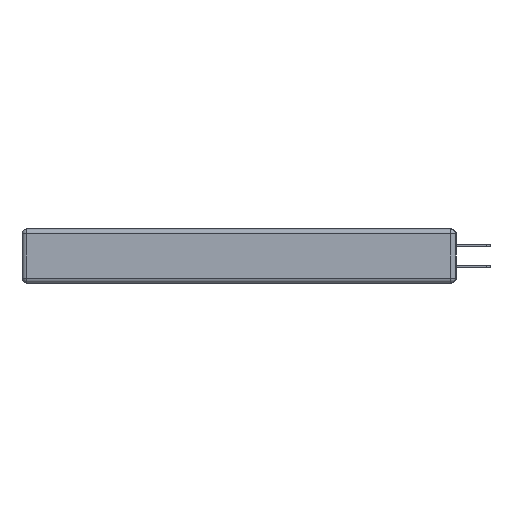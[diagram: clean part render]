
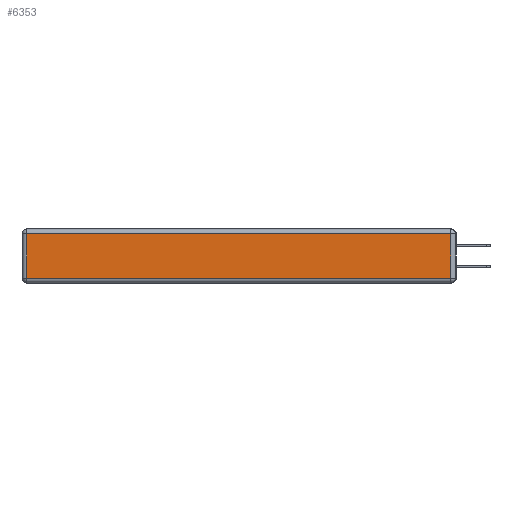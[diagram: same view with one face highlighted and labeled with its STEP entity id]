
A CAD part, left-side view. The second image highlights one B-rep face of the part: STEP entity #6353.
In plain terms, the highlighted planar face has unit normal (-1, 0, 0).
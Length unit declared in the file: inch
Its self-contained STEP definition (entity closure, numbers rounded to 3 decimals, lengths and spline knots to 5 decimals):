
#1629 = EDGE_CURVE ( 'NONE', #18775, #14641, #4996, .T. ) ;
#1783 = AXIS2_PLACEMENT_3D ( 'NONE', #25220, #7369, #4642 ) ;
#2307 = LINE ( 'NONE', #11097, #9630 ) ;
#4642 = DIRECTION ( 'NONE',  ( 0., 0., 1. ) ) ;
#4765 = VECTOR ( 'NONE', #14513, 39.37008 ) ;
#4897 = ORIENTED_EDGE ( 'NONE', *, *, #17855, .T. ) ;
#4996 = LINE ( 'NONE', #10354, #7459 ) ;
#6353 = ADVANCED_FACE ( 'NONE', ( #17303 ), #22908, .T. ) ;
#6403 = LINE ( 'NONE', #9118, #4765 ) ;
#7369 = DIRECTION ( 'NONE',  ( -1., 0., 0. ) ) ;
#7459 = VECTOR ( 'NONE', #23072, 39.37008 ) ;
#8377 = LINE ( 'NONE', #27787, #30769 ) ;
#8477 = CARTESIAN_POINT ( 'NONE',  ( 0., 0.03, -0.03 ) ) ;
#9118 = CARTESIAN_POINT ( 'NONE',  ( 0., 2.72, -0.343 ) ) ;
#9513 = ORIENTED_EDGE ( 'NONE', *, *, #1629, .T. ) ;
#9630 = VECTOR ( 'NONE', #29407, 39.37008 ) ;
#9848 = CARTESIAN_POINT ( 'NONE',  ( 0., 2.72, -0.03 ) ) ;
#10038 = DIRECTION ( 'NONE',  ( 0., -1., 0. ) ) ;
#10354 = CARTESIAN_POINT ( 'NONE',  ( 0., 0.03, -0.343 ) ) ;
#10430 = CARTESIAN_POINT ( 'NONE',  ( 0., 0.03, -0.313 ) ) ;
#11097 = CARTESIAN_POINT ( 'NONE',  ( 0., 2.75, -0.03 ) ) ;
#13519 = EDGE_LOOP ( 'NONE', ( #4897, #9513, #23806, #16419 ) ) ;
#14513 = DIRECTION ( 'NONE',  ( 0., 0., -1. ) ) ;
#14641 = VERTEX_POINT ( 'NONE', #8477 ) ;
#16419 = ORIENTED_EDGE ( 'NONE', *, *, #23112, .T. ) ;
#17303 = FACE_OUTER_BOUND ( 'NONE', #13519, .T. ) ;
#17855 = EDGE_CURVE ( 'NONE', #26149, #18775, #8377, .T. ) ;
#18775 = VERTEX_POINT ( 'NONE', #10430 ) ;
#19156 = CARTESIAN_POINT ( 'NONE',  ( 0., 2.72, -0.313 ) ) ;
#20153 = VERTEX_POINT ( 'NONE', #9848 ) ;
#22908 = PLANE ( 'NONE',  #1783 ) ;
#23072 = DIRECTION ( 'NONE',  ( 0., 0., 1. ) ) ;
#23112 = EDGE_CURVE ( 'NONE', #20153, #26149, #6403, .T. ) ;
#23806 = ORIENTED_EDGE ( 'NONE', *, *, #32015, .T. ) ;
#25220 = CARTESIAN_POINT ( 'NONE',  ( 0., 0., -0.343 ) ) ;
#26149 = VERTEX_POINT ( 'NONE', #19156 ) ;
#27787 = CARTESIAN_POINT ( 'NONE',  ( 0., 0., -0.313 ) ) ;
#29407 = DIRECTION ( 'NONE',  ( 0., 1., 0. ) ) ;
#30769 = VECTOR ( 'NONE', #10038, 39.37008 ) ;
#32015 = EDGE_CURVE ( 'NONE', #14641, #20153, #2307, .T. ) ;
